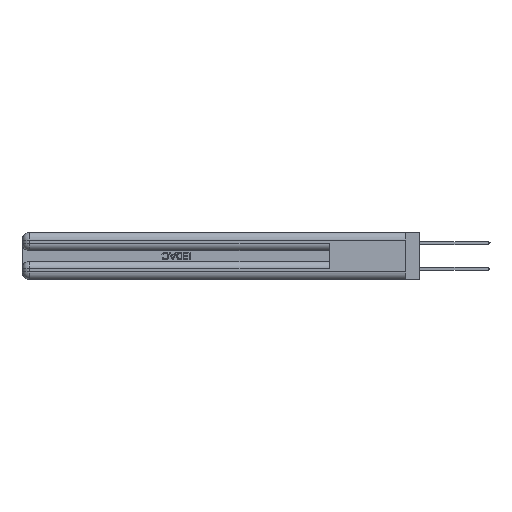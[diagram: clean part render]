
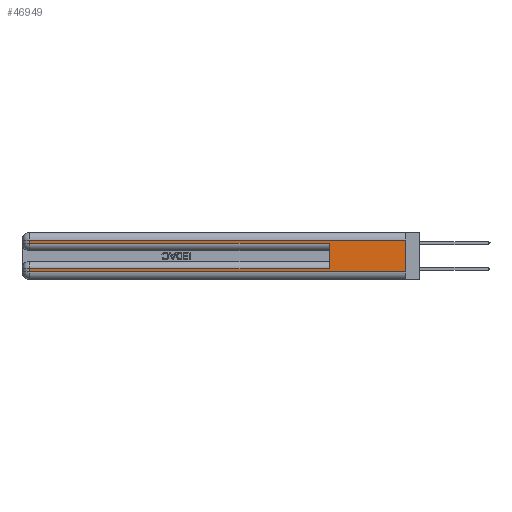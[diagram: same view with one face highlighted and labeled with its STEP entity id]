
A CAD part, left-side view. The second image highlights one B-rep face of the part: STEP entity #46949.
In plain terms, the highlighted planar face has unit normal (-1, 0, 0).
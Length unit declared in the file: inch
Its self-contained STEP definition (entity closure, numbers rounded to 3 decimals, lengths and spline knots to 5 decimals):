
#22 = DIRECTION ( 'NONE',  ( 1., 0., 0. ) ) ;
#700 = CARTESIAN_POINT ( 'NONE',  ( 0., 2.94, 0.085 ) ) ;
#1134 = VECTOR ( 'NONE', #39161, 39.37008 ) ;
#1296 = VECTOR ( 'NONE', #34574, 39.37008 ) ;
#2161 = ORIENTED_EDGE ( 'NONE', *, *, #32207, .T. ) ;
#3680 = VECTOR ( 'NONE', #46158, 39.37008 ) ;
#4130 = CARTESIAN_POINT ( 'NONE',  ( 0., 2.94, 0.31 ) ) ;
#4831 = LINE ( 'NONE', #35448, #3680 ) ;
#4840 = CARTESIAN_POINT ( 'NONE',  ( 0., 0., 0.31 ) ) ;
#5025 = LINE ( 'NONE', #35507, #45675 ) ;
#7285 = LINE ( 'NONE', #4840, #42756 ) ;
#7474 = CARTESIAN_POINT ( 'NONE',  ( 0., 0., 0.285 ) ) ;
#7484 = DIRECTION ( 'NONE',  ( 0., 0., -1. ) ) ;
#8166 = EDGE_CURVE ( 'NONE', #13057, #26764, #4831, .T. ) ;
#10707 = ORIENTED_EDGE ( 'NONE', *, *, #11798, .T. ) ;
#10750 = FACE_OUTER_BOUND ( 'NONE', #45296, .T. ) ;
#11028 = CARTESIAN_POINT ( 'NONE',  ( 0., 0.6, 0.285 ) ) ;
#11188 = LINE ( 'NONE', #30683, #1296 ) ;
#11510 = LINE ( 'NONE', #47558, #47001 ) ;
#11683 = VECTOR ( 'NONE', #38033, 39.37008 ) ;
#11798 = EDGE_CURVE ( 'NONE', #21673, #13057, #40718, .T. ) ;
#12167 = LINE ( 'NONE', #7474, #24334 ) ;
#12602 = EDGE_CURVE ( 'NONE', #25530, #23881, #11510, .T. ) ;
#13057 = VERTEX_POINT ( 'NONE', #22138 ) ;
#15078 = PLANE ( 'NONE',  #30254 ) ;
#15201 = EDGE_CURVE ( 'NONE', #18930, #26764, #21545, .T. ) ;
#17315 = DIRECTION ( 'NONE',  ( 0., 0., 1. ) ) ;
#18048 = EDGE_CURVE ( 'NONE', #38812, #32913, #5025, .T. ) ;
#18930 = VERTEX_POINT ( 'NONE', #32987 ) ;
#19469 = EDGE_CURVE ( 'NONE', #18930, #38812, #7285, .T. ) ;
#20263 = CARTESIAN_POINT ( 'NONE',  ( 0., 2.94, 0.37 ) ) ;
#21374 = ORIENTED_EDGE ( 'NONE', *, *, #19469, .T. ) ;
#21545 = LINE ( 'NONE', #23331, #11683 ) ;
#21673 = VERTEX_POINT ( 'NONE', #700 ) ;
#22027 = CARTESIAN_POINT ( 'NONE',  ( 0., 0., 0.37 ) ) ;
#22138 = CARTESIAN_POINT ( 'NONE',  ( 0., 2.94, 0.06 ) ) ;
#23331 = CARTESIAN_POINT ( 'NONE',  ( 0., 0., 0.37 ) ) ;
#23881 = VERTEX_POINT ( 'NONE', #11028 ) ;
#24334 = VECTOR ( 'NONE', #40114, 39.37008 ) ;
#25530 = VERTEX_POINT ( 'NONE', #43355 ) ;
#26457 = ORIENTED_EDGE ( 'NONE', *, *, #8166, .T. ) ;
#26764 = VERTEX_POINT ( 'NONE', #45166 ) ;
#29410 = ORIENTED_EDGE ( 'NONE', *, *, #12602, .F. ) ;
#30254 = AXIS2_PLACEMENT_3D ( 'NONE', #22027, #22, #7484 ) ;
#30683 = CARTESIAN_POINT ( 'NONE',  ( 0., 0., 0.085 ) ) ;
#32207 = EDGE_CURVE ( 'NONE', #32913, #23881, #12167, .T. ) ;
#32913 = VERTEX_POINT ( 'NONE', #40968 ) ;
#32987 = CARTESIAN_POINT ( 'NONE',  ( 0., 0., 0.31 ) ) ;
#34574 = DIRECTION ( 'NONE',  ( 0., 1., 0. ) ) ;
#35448 = CARTESIAN_POINT ( 'NONE',  ( 0., 0., 0.06 ) ) ;
#35507 = CARTESIAN_POINT ( 'NONE',  ( 0., 2.94, 0.37 ) ) ;
#38033 = DIRECTION ( 'NONE',  ( 0., 0., -1. ) ) ;
#38812 = VERTEX_POINT ( 'NONE', #4130 ) ;
#39161 = DIRECTION ( 'NONE',  ( 0., 0., -1. ) ) ;
#40114 = DIRECTION ( 'NONE',  ( 0., -1., 0. ) ) ;
#40566 = ORIENTED_EDGE ( 'NONE', *, *, #41949, .T. ) ;
#40718 = LINE ( 'NONE', #20263, #1134 ) ;
#40968 = CARTESIAN_POINT ( 'NONE',  ( 0., 2.94, 0.285 ) ) ;
#41949 = EDGE_CURVE ( 'NONE', #25530, #21673, #11188, .T. ) ;
#42426 = ORIENTED_EDGE ( 'NONE', *, *, #18048, .T. ) ;
#42756 = VECTOR ( 'NONE', #44209, 39.37008 ) ;
#43183 = DIRECTION ( 'NONE',  ( 0., 0., -1. ) ) ;
#43355 = CARTESIAN_POINT ( 'NONE',  ( 0., 0.6, 0.085 ) ) ;
#43657 = ORIENTED_EDGE ( 'NONE', *, *, #15201, .F. ) ;
#44209 = DIRECTION ( 'NONE',  ( 0., 1., 0. ) ) ;
#45166 = CARTESIAN_POINT ( 'NONE',  ( 0., 0., 0.06 ) ) ;
#45296 = EDGE_LOOP ( 'NONE', ( #43657, #21374, #42426, #2161, #29410, #40566, #10707, #26457 ) ) ;
#45675 = VECTOR ( 'NONE', #43183, 39.37008 ) ;
#46158 = DIRECTION ( 'NONE',  ( 0., -1., 0. ) ) ;
#46949 = ADVANCED_FACE ( 'NONE', ( #10750 ), #15078, .F. ) ;
#47001 = VECTOR ( 'NONE', #17315, 39.37008 ) ;
#47558 = CARTESIAN_POINT ( 'NONE',  ( 0., 0.6, 0.145 ) ) ;
